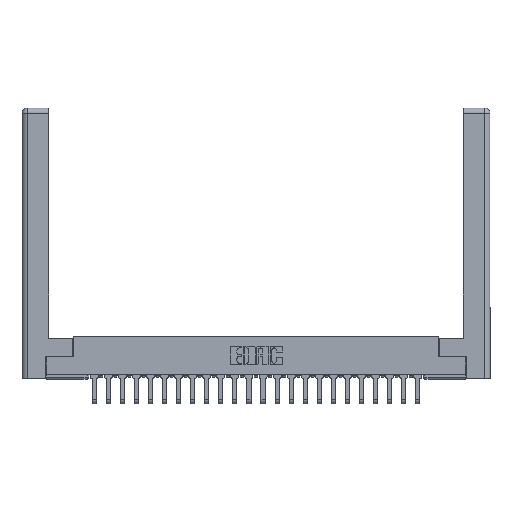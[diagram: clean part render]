
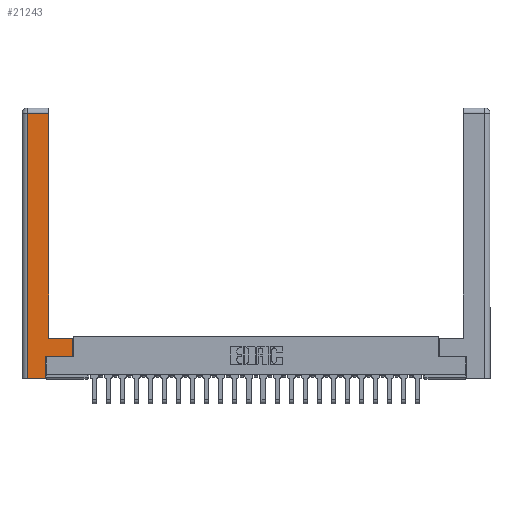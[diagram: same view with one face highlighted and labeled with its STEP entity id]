
A CAD part, top view. The second image highlights one B-rep face of the part: STEP entity #21243.
In plain terms, the highlighted planar face has unit normal (0, 0, 1).
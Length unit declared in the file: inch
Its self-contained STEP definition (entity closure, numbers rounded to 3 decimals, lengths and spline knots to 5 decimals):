
#282 = CARTESIAN_POINT ( 'NONE',  ( 0.265, 0., 0. ) ) ;
#460 = CARTESIAN_POINT ( 'NONE',  ( 0.0615, 0., 0. ) ) ;
#479 = LINE ( 'NONE', #460, #1152 ) ;
#489 = ORIENTED_EDGE ( 'NONE', *, *, #22569, .T. ) ;
#513 = ORIENTED_EDGE ( 'NONE', *, *, #8532, .T. ) ;
#739 = DIRECTION ( 'NONE',  ( -1., 0., 0. ) ) ;
#821 = VECTOR ( 'NONE', #14155, 39.37008 ) ;
#1152 = VECTOR ( 'NONE', #17700, 39.37008 ) ;
#1515 = CARTESIAN_POINT ( 'NONE',  ( 0.0615, 2.94, 0. ) ) ;
#2539 = LINE ( 'NONE', #21293, #5827 ) ;
#2888 = VERTEX_POINT ( 'NONE', #15674 ) ;
#3049 = CARTESIAN_POINT ( 'NONE',  ( 0.0615, 0., 0. ) ) ;
#3567 = VERTEX_POINT ( 'NONE', #282 ) ;
#3801 = DIRECTION ( 'NONE',  ( 0., 1., 0. ) ) ;
#3967 = LINE ( 'NONE', #16237, #20297 ) ;
#4260 = LINE ( 'NONE', #10071, #10551 ) ;
#4844 = ORIENTED_EDGE ( 'NONE', *, *, #8259, .T. ) ;
#5280 = LINE ( 'NONE', #1515, #27352 ) ;
#5827 = VECTOR ( 'NONE', #21105, 39.37008 ) ;
#5988 = VERTEX_POINT ( 'NONE', #17611 ) ;
#7055 = DIRECTION ( 'NONE',  ( 0., 1., 0. ) ) ;
#7071 = LINE ( 'NONE', #9157, #10032 ) ;
#7891 = LINE ( 'NONE', #17189, #27637 ) ;
#8259 = EDGE_CURVE ( 'NONE', #27259, #3567, #14157, .T. ) ;
#8532 = EDGE_CURVE ( 'NONE', #5988, #27259, #479, .T. ) ;
#9157 = CARTESIAN_POINT ( 'NONE',  ( 0.565, 0.45, 0. ) ) ;
#9160 = ORIENTED_EDGE ( 'NONE', *, *, #18768, .T. ) ;
#10032 = VECTOR ( 'NONE', #7055, 39.37008 ) ;
#10071 = CARTESIAN_POINT ( 'NONE',  ( 0.295, 0.45, 0. ) ) ;
#10551 = VECTOR ( 'NONE', #17287, 39.37008 ) ;
#10940 = FACE_OUTER_BOUND ( 'NONE', #26005, .T. ) ;
#11371 = VERTEX_POINT ( 'NONE', #12502 ) ;
#12502 = CARTESIAN_POINT ( 'NONE',  ( 0.265, 0.245, 0. ) ) ;
#12551 = ORIENTED_EDGE ( 'NONE', *, *, #16027, .T. ) ;
#13293 = CARTESIAN_POINT ( 'NONE',  ( 0., 0., 0. ) ) ;
#14155 = DIRECTION ( 'NONE',  ( 1., 0., 0. ) ) ;
#14157 = LINE ( 'NONE', #14247, #821 ) ;
#14247 = CARTESIAN_POINT ( 'NONE',  ( 0.265, 0., 0. ) ) ;
#14372 = VERTEX_POINT ( 'NONE', #18767 ) ;
#15674 = CARTESIAN_POINT ( 'NONE',  ( 0.295, 0.45, 0. ) ) ;
#15979 = EDGE_CURVE ( 'NONE', #2888, #27600, #7891, .T. ) ;
#16027 = EDGE_CURVE ( 'NONE', #21278, #2888, #4260, .T. ) ;
#16227 = ORIENTED_EDGE ( 'NONE', *, *, #26432, .T. ) ;
#16237 = CARTESIAN_POINT ( 'NONE',  ( 0.265, 0.245, 0. ) ) ;
#16512 = AXIS2_PLACEMENT_3D ( 'NONE', #13293, #22168, #739 ) ;
#16515 = DIRECTION ( 'NONE',  ( 0., 1., 0. ) ) ;
#17189 = CARTESIAN_POINT ( 'NONE',  ( 0.295, 3., 0. ) ) ;
#17287 = DIRECTION ( 'NONE',  ( -1., 0., 0. ) ) ;
#17611 = CARTESIAN_POINT ( 'NONE',  ( 0.0615, 2.94, 0. ) ) ;
#17700 = DIRECTION ( 'NONE',  ( 0., -1., 0. ) ) ;
#18767 = CARTESIAN_POINT ( 'NONE',  ( 0.565, 0.245, 0. ) ) ;
#18768 = EDGE_CURVE ( 'NONE', #14372, #21278, #7071, .T. ) ;
#19848 = CARTESIAN_POINT ( 'NONE',  ( 0.565, 0.45, 0. ) ) ;
#20297 = VECTOR ( 'NONE', #16515, 39.37008 ) ;
#21105 = DIRECTION ( 'NONE',  ( 1., 0., 0. ) ) ;
#21243 = ADVANCED_FACE ( 'NONE', ( #10940 ), #23789, .F. ) ;
#21278 = VERTEX_POINT ( 'NONE', #19848 ) ;
#21293 = CARTESIAN_POINT ( 'NONE',  ( 0.565, 0.245, 0. ) ) ;
#22168 = DIRECTION ( 'NONE',  ( 0., 0., -1. ) ) ;
#22569 = EDGE_CURVE ( 'NONE', #3567, #11371, #3967, .T. ) ;
#23517 = CARTESIAN_POINT ( 'NONE',  ( 0.295, 2.94, 0. ) ) ;
#23789 = PLANE ( 'NONE',  #16512 ) ;
#24152 = EDGE_CURVE ( 'NONE', #11371, #14372, #2539, .T. ) ;
#24772 = ORIENTED_EDGE ( 'NONE', *, *, #15979, .T. ) ;
#24943 = DIRECTION ( 'NONE',  ( -1., 0., 0. ) ) ;
#25726 = ORIENTED_EDGE ( 'NONE', *, *, #24152, .T. ) ;
#26005 = EDGE_LOOP ( 'NONE', ( #24772, #16227, #513, #4844, #489, #25726, #9160, #12551 ) ) ;
#26432 = EDGE_CURVE ( 'NONE', #27600, #5988, #5280, .T. ) ;
#27259 = VERTEX_POINT ( 'NONE', #3049 ) ;
#27352 = VECTOR ( 'NONE', #24943, 39.37008 ) ;
#27600 = VERTEX_POINT ( 'NONE', #23517 ) ;
#27637 = VECTOR ( 'NONE', #3801, 39.37008 ) ;
